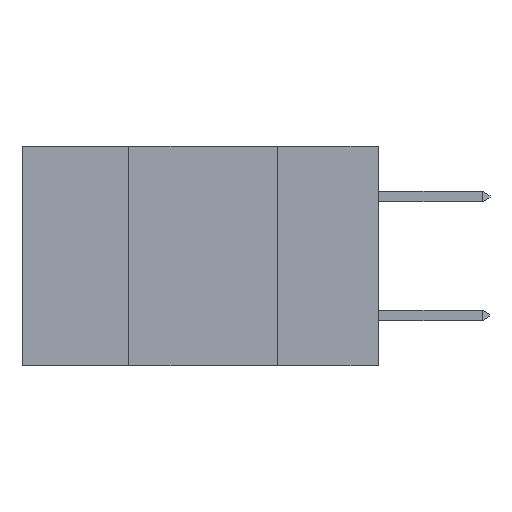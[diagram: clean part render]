
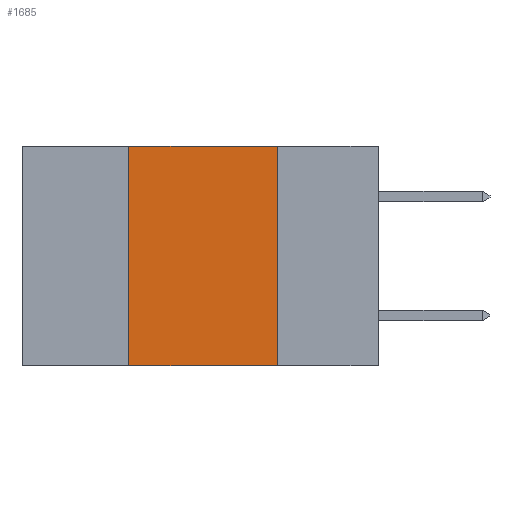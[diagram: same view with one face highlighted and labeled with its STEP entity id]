
A CAD part, left-side view. The second image highlights one B-rep face of the part: STEP entity #1685.
In plain terms, the highlighted planar face has unit normal (-1, 0, 0).
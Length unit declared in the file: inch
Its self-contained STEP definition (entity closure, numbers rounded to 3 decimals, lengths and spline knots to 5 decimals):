
#34 = EDGE_LOOP ( 'NONE', ( #1798, #1897, #2127, #2214 ) ) ;
#309 = DIRECTION ( 'NONE',  ( 0., -1., 0. ) ) ;
#1685 = ADVANCED_FACE ( 'NONE', ( #9321 ), #2649, .F. ) ;
#1798 = ORIENTED_EDGE ( 'NONE', *, *, #7527, .F. ) ;
#1800 = DIRECTION ( 'NONE',  ( 0., -1., 0. ) ) ;
#1897 = ORIENTED_EDGE ( 'NONE', *, *, #8194, .F. ) ;
#2011 = CARTESIAN_POINT ( 'NONE',  ( 0., 0.6, 0. ) ) ;
#2127 = ORIENTED_EDGE ( 'NONE', *, *, #5663, .F. ) ;
#2214 = ORIENTED_EDGE ( 'NONE', *, *, #4726, .T. ) ;
#2649 = PLANE ( 'NONE',  #3711 ) ;
#3369 = LINE ( 'NONE', #5708, #6950 ) ;
#3537 = VERTEX_POINT ( 'NONE', #8958 ) ;
#3711 = AXIS2_PLACEMENT_3D ( 'NONE', #6754, #8224, #4994 ) ;
#4078 = CARTESIAN_POINT ( 'NONE',  ( 0., 0.42, 0. ) ) ;
#4242 = DIRECTION ( 'NONE',  ( 0., 0., 1. ) ) ;
#4265 = CARTESIAN_POINT ( 'NONE',  ( 0., 0.6, -0.37 ) ) ;
#4726 = EDGE_CURVE ( 'NONE', #3537, #5497, #5676, .T. ) ;
#4994 = DIRECTION ( 'NONE',  ( 0., 0., -1. ) ) ;
#5130 = VECTOR ( 'NONE', #4242, 39.37008 ) ;
#5497 = VERTEX_POINT ( 'NONE', #8240 ) ;
#5590 = DIRECTION ( 'NONE',  ( 0., 0., -1. ) ) ;
#5663 = EDGE_CURVE ( 'NONE', #3537, #5990, #6989, .T. ) ;
#5676 = LINE ( 'NONE', #4265, #8652 ) ;
#5708 = CARTESIAN_POINT ( 'NONE',  ( 0., 0.17, 0. ) ) ;
#5990 = VERTEX_POINT ( 'NONE', #4078 ) ;
#6167 = VERTEX_POINT ( 'NONE', #8580 ) ;
#6583 = CARTESIAN_POINT ( 'NONE',  ( 0., 0.42, 0. ) ) ;
#6754 = CARTESIAN_POINT ( 'NONE',  ( 0., 0.6, 0. ) ) ;
#6950 = VECTOR ( 'NONE', #5590, 39.37008 ) ;
#6989 = LINE ( 'NONE', #6583, #5130 ) ;
#7148 = VECTOR ( 'NONE', #1800, 39.37008 ) ;
#7363 = LINE ( 'NONE', #2011, #7148 ) ;
#7527 = EDGE_CURVE ( 'NONE', #6167, #5497, #3369, .T. ) ;
#8194 = EDGE_CURVE ( 'NONE', #5990, #6167, #7363, .T. ) ;
#8224 = DIRECTION ( 'NONE',  ( 1., 0., 0. ) ) ;
#8240 = CARTESIAN_POINT ( 'NONE',  ( 0., 0.17, -0.37 ) ) ;
#8580 = CARTESIAN_POINT ( 'NONE',  ( 0., 0.17, 0. ) ) ;
#8652 = VECTOR ( 'NONE', #309, 39.37008 ) ;
#8958 = CARTESIAN_POINT ( 'NONE',  ( 0., 0.42, -0.37 ) ) ;
#9321 = FACE_OUTER_BOUND ( 'NONE', #34, .T. ) ;
